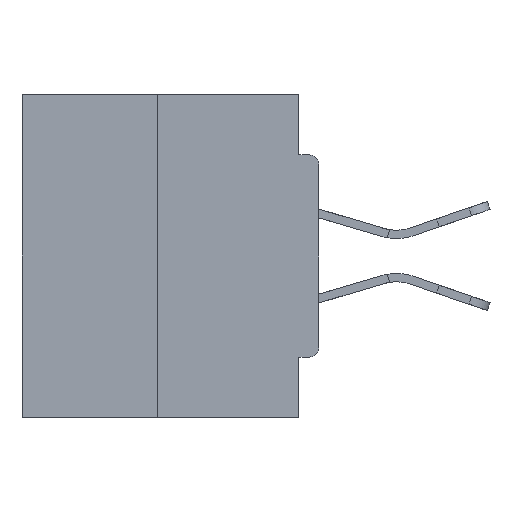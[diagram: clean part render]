
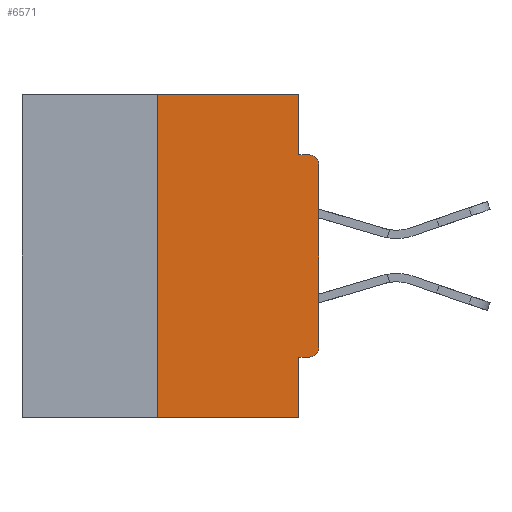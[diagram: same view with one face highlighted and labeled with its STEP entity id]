
A CAD part, left-side view. The second image highlights one B-rep face of the part: STEP entity #6571.
In plain terms, the highlighted planar face has unit normal (-1, 0, 0).
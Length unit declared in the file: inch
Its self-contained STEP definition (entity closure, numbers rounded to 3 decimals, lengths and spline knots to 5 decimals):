
#339 = LINE ( 'NONE', #9842, #18488 ) ;
#340 = AXIS2_PLACEMENT_3D ( 'NONE', #11141, #1052, #15052 ) ;
#660 = CARTESIAN_POINT ( 'NONE',  ( 0., 0.031, 0. ) ) ;
#1052 = DIRECTION ( 'NONE',  ( 1., 0., 0. ) ) ;
#1254 = CARTESIAN_POINT ( 'NONE',  ( 0., 0.46, -0.5 ) ) ;
#2401 = VECTOR ( 'NONE', #31153, 39.37008 ) ;
#2605 = ORIENTED_EDGE ( 'NONE', *, *, #4599, .F. ) ;
#3521 = VERTEX_POINT ( 'NONE', #660 ) ;
#3531 = CARTESIAN_POINT ( 'NONE',  ( 0., 0.25, 0. ) ) ;
#3742 = LINE ( 'NONE', #16330, #27858 ) ;
#4142 = CARTESIAN_POINT ( 'NONE',  ( 0., 0.031, -0.4065 ) ) ;
#4599 = EDGE_CURVE ( 'NONE', #5193, #24234, #339, .T. ) ;
#4644 = DIRECTION ( 'NONE',  ( 0., 1., 0. ) ) ;
#5193 = VERTEX_POINT ( 'NONE', #30685 ) ;
#5227 = ORIENTED_EDGE ( 'NONE', *, *, #6285, .F. ) ;
#5262 = VERTEX_POINT ( 'NONE', #5577 ) ;
#5577 = CARTESIAN_POINT ( 'NONE',  ( 0., 0.031, -0.5 ) ) ;
#6094 = EDGE_CURVE ( 'NONE', #31463, #5262, #17117, .T. ) ;
#6285 = EDGE_CURVE ( 'NONE', #31463, #22427, #3742, .T. ) ;
#6398 = EDGE_CURVE ( 'NONE', #19176, #28071, #14602, .T. ) ;
#6571 = ADVANCED_FACE ( 'NONE', ( #26912 ), #22097, .F. ) ;
#6898 = DIRECTION ( 'NONE',  ( 0., -1., 0. ) ) ;
#6914 = EDGE_CURVE ( 'NONE', #5193, #25062, #23004, .T. ) ;
#8492 = CARTESIAN_POINT ( 'NONE',  ( 0., 0.031, -0.0935 ) ) ;
#8939 = CARTESIAN_POINT ( 'NONE',  ( 0., 0.031, -0.5 ) ) ;
#9261 = VECTOR ( 'NONE', #13793, 39.37008 ) ;
#9569 = CARTESIAN_POINT ( 'NONE',  ( 0., 0.015, -0.1085 ) ) ;
#9842 = CARTESIAN_POINT ( 'NONE',  ( 0., 0., -0.4065 ) ) ;
#10548 = CARTESIAN_POINT ( 'NONE',  ( 0., 0.25, -0.5 ) ) ;
#11121 = CARTESIAN_POINT ( 'NONE',  ( 0., 0.015, -0.0935 ) ) ;
#11141 = CARTESIAN_POINT ( 'NONE',  ( 0., 0.46, 0. ) ) ;
#11813 = CARTESIAN_POINT ( 'NONE',  ( 0., 0.031, 0. ) ) ;
#13793 = DIRECTION ( 'NONE',  ( 0., 0., 1. ) ) ;
#14108 = VECTOR ( 'NONE', #34555, 39.37008 ) ;
#14196 = EDGE_CURVE ( 'NONE', #21245, #28071, #32682, .T. ) ;
#14602 = LINE ( 'NONE', #28766, #14108 ) ;
#14724 = ORIENTED_EDGE ( 'NONE', *, *, #14196, .T. ) ;
#15052 = DIRECTION ( 'NONE',  ( 0., 0., -1. ) ) ;
#15103 = ORIENTED_EDGE ( 'NONE', *, *, #33105, .T. ) ;
#15485 = ORIENTED_EDGE ( 'NONE', *, *, #6094, .T. ) ;
#15736 = ORIENTED_EDGE ( 'NONE', *, *, #33434, .F. ) ;
#16330 = CARTESIAN_POINT ( 'NONE',  ( 0., 0.25, 0. ) ) ;
#16463 = AXIS2_PLACEMENT_3D ( 'NONE', #9569, #28858, #18167 ) ;
#16582 = CARTESIAN_POINT ( 'NONE',  ( 0., 0., 0. ) ) ;
#16938 = EDGE_CURVE ( 'NONE', #3521, #19176, #35311, .T. ) ;
#17117 = LINE ( 'NONE', #1254, #2401 ) ;
#17788 = CARTESIAN_POINT ( 'NONE',  ( 0., 0.46, 0. ) ) ;
#18167 = DIRECTION ( 'NONE',  ( 0., 0., -1. ) ) ;
#18488 = VECTOR ( 'NONE', #4644, 39.37008 ) ;
#18647 = ORIENTED_EDGE ( 'NONE', *, *, #19432, .F. ) ;
#18908 = VECTOR ( 'NONE', #28180, 39.37008 ) ;
#19130 = ORIENTED_EDGE ( 'NONE', *, *, #6914, .T. ) ;
#19176 = VERTEX_POINT ( 'NONE', #8492 ) ;
#19432 = EDGE_CURVE ( 'NONE', #22427, #3521, #22182, .T. ) ;
#20732 = ORIENTED_EDGE ( 'NONE', *, *, #16938, .F. ) ;
#21245 = VERTEX_POINT ( 'NONE', #26986 ) ;
#21850 = AXIS2_PLACEMENT_3D ( 'NONE', #27454, #30202, #30576 ) ;
#22097 = PLANE ( 'NONE',  #340 ) ;
#22182 = LINE ( 'NONE', #17788, #32992 ) ;
#22427 = VERTEX_POINT ( 'NONE', #3531 ) ;
#23004 = CIRCLE ( 'NONE', #21850, 0.015 ) ;
#23919 = LINE ( 'NONE', #16582, #9261 ) ;
#24234 = VERTEX_POINT ( 'NONE', #4142 ) ;
#25062 = VERTEX_POINT ( 'NONE', #33486 ) ;
#25856 = ORIENTED_EDGE ( 'NONE', *, *, #6398, .F. ) ;
#26912 = FACE_OUTER_BOUND ( 'NONE', #29031, .T. ) ;
#26986 = CARTESIAN_POINT ( 'NONE',  ( 0., 0., -0.1085 ) ) ;
#27454 = CARTESIAN_POINT ( 'NONE',  ( 0., 0.015, -0.3915 ) ) ;
#27858 = VECTOR ( 'NONE', #32901, 39.37008 ) ;
#28071 = VERTEX_POINT ( 'NONE', #11121 ) ;
#28180 = DIRECTION ( 'NONE',  ( 0., 0., -1. ) ) ;
#28766 = CARTESIAN_POINT ( 'NONE',  ( 0., 0., -0.0935 ) ) ;
#28858 = DIRECTION ( 'NONE',  ( -1., 0., 0. ) ) ;
#29031 = EDGE_LOOP ( 'NONE', ( #18647, #5227, #15485, #15736, #2605, #19130, #15103, #14724, #25856, #20732 ) ) ;
#30202 = DIRECTION ( 'NONE',  ( -1., 0., 0. ) ) ;
#30377 = LINE ( 'NONE', #8939, #34736 ) ;
#30576 = DIRECTION ( 'NONE',  ( 0., 0., -1. ) ) ;
#30685 = CARTESIAN_POINT ( 'NONE',  ( 0., 0.015, -0.4065 ) ) ;
#31153 = DIRECTION ( 'NONE',  ( 0., -1., 0. ) ) ;
#31249 = DIRECTION ( 'NONE',  ( 0., 0., -1. ) ) ;
#31463 = VERTEX_POINT ( 'NONE', #10548 ) ;
#32682 = CIRCLE ( 'NONE', #16463, 0.015 ) ;
#32901 = DIRECTION ( 'NONE',  ( 0., 0., 1. ) ) ;
#32992 = VECTOR ( 'NONE', #6898, 39.37008 ) ;
#33105 = EDGE_CURVE ( 'NONE', #25062, #21245, #23919, .T. ) ;
#33434 = EDGE_CURVE ( 'NONE', #24234, #5262, #30377, .T. ) ;
#33486 = CARTESIAN_POINT ( 'NONE',  ( 0., 0., -0.3915 ) ) ;
#34555 = DIRECTION ( 'NONE',  ( 0., -1., 0. ) ) ;
#34736 = VECTOR ( 'NONE', #31249, 39.37008 ) ;
#35311 = LINE ( 'NONE', #11813, #18908 ) ;
